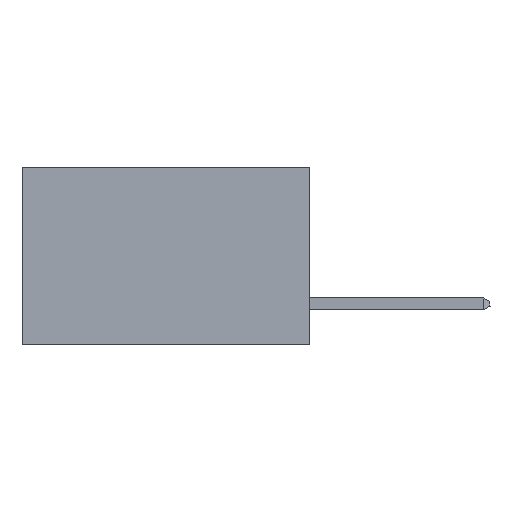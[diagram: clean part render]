
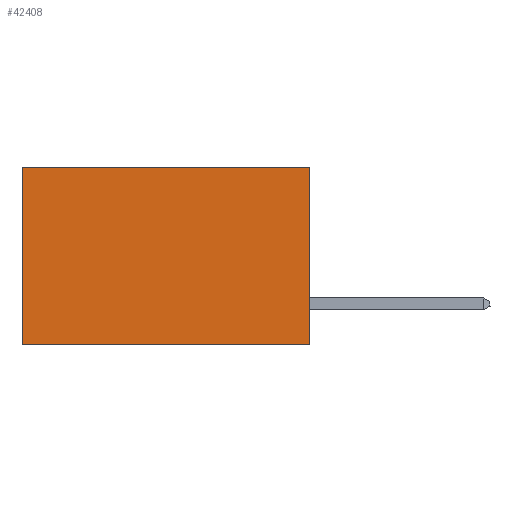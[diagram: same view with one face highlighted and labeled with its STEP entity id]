
A CAD part, left-side view. The second image highlights one B-rep face of the part: STEP entity #42408.
In plain terms, the highlighted planar face has unit normal (-1, 0, 0).
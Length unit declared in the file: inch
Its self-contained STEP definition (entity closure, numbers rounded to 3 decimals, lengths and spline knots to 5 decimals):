
#656 = VECTOR ( 'NONE', #6735, 39.37008 ) ;
#1305 = EDGE_CURVE ( 'NONE', #13086, #47959, #43138, .T. ) ;
#1307 = EDGE_CURVE ( 'NONE', #47001, #31623, #1512, .T. ) ;
#1512 = LINE ( 'NONE', #4510, #29469 ) ;
#3554 = ORIENTED_EDGE ( 'NONE', *, *, #1305, .F. ) ;
#3705 = CARTESIAN_POINT ( 'NONE',  ( 0.2875, 0., 0. ) ) ;
#4203 = DIRECTION ( 'NONE',  ( 0., 1., 0. ) ) ;
#4510 = CARTESIAN_POINT ( 'NONE',  ( 0.2875, 0., 0. ) ) ;
#6735 = DIRECTION ( 'NONE',  ( 0., 0., -1. ) ) ;
#8326 = CARTESIAN_POINT ( 'NONE',  ( 0.2875, 0., -0.37 ) ) ;
#9328 = ORIENTED_EDGE ( 'NONE', *, *, #26679, .F. ) ;
#12304 = CARTESIAN_POINT ( 'NONE',  ( 0.2875, 0., 0. ) ) ;
#13086 = VERTEX_POINT ( 'NONE', #31501 ) ;
#14866 = ORIENTED_EDGE ( 'NONE', *, *, #39956, .T. ) ;
#16373 = FACE_OUTER_BOUND ( 'NONE', #20043, .T. ) ;
#17593 = CARTESIAN_POINT ( 'NONE',  ( 0.2875, 0.6, -0.37 ) ) ;
#18888 = VECTOR ( 'NONE', #4203, 39.37008 ) ;
#20043 = EDGE_LOOP ( 'NONE', ( #14866, #3554, #9328, #24114 ) ) ;
#20224 = VECTOR ( 'NONE', #21479, 39.37008 ) ;
#21479 = DIRECTION ( 'NONE',  ( 0., 0., -1. ) ) ;
#24114 = ORIENTED_EDGE ( 'NONE', *, *, #1307, .T. ) ;
#24299 = CARTESIAN_POINT ( 'NONE',  ( 0.2875, 0.6, 0. ) ) ;
#24713 = DIRECTION ( 'NONE',  ( 0., 0., -1. ) ) ;
#24887 = DIRECTION ( 'NONE',  ( 1., 0., 0. ) ) ;
#26679 = EDGE_CURVE ( 'NONE', #47001, #13086, #33437, .T. ) ;
#28332 = PLANE ( 'NONE',  #40893 ) ;
#28700 = CARTESIAN_POINT ( 'NONE',  ( 0.2875, 0.6, 0. ) ) ;
#29469 = VECTOR ( 'NONE', #31019, 39.37008 ) ;
#31019 = DIRECTION ( 'NONE',  ( 0., 1., 0. ) ) ;
#31501 = CARTESIAN_POINT ( 'NONE',  ( 0.2875, 0., -0.37 ) ) ;
#31623 = VERTEX_POINT ( 'NONE', #24299 ) ;
#32679 = CARTESIAN_POINT ( 'NONE',  ( 0.2875, 0., 0. ) ) ;
#33437 = LINE ( 'NONE', #3705, #656 ) ;
#39956 = EDGE_CURVE ( 'NONE', #31623, #47959, #48172, .T. ) ;
#40893 = AXIS2_PLACEMENT_3D ( 'NONE', #32679, #24887, #24713 ) ;
#42408 = ADVANCED_FACE ( 'NONE', ( #16373 ), #28332, .F. ) ;
#43138 = LINE ( 'NONE', #8326, #18888 ) ;
#47001 = VERTEX_POINT ( 'NONE', #12304 ) ;
#47959 = VERTEX_POINT ( 'NONE', #17593 ) ;
#48172 = LINE ( 'NONE', #28700, #20224 ) ;
